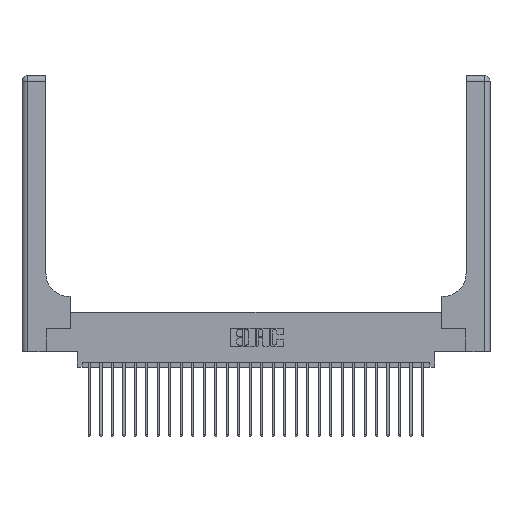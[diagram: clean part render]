
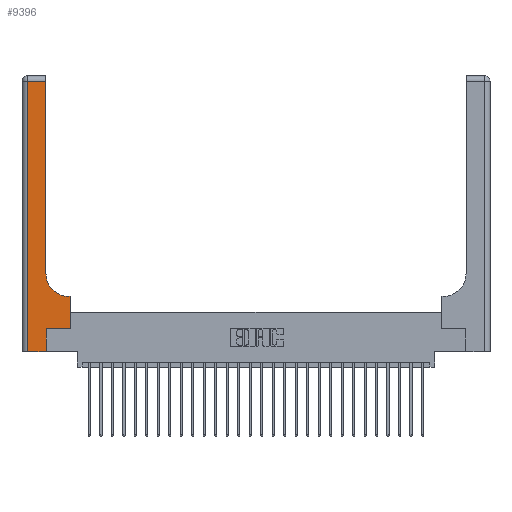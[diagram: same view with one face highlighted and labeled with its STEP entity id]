
A CAD part, top view. The second image highlights one B-rep face of the part: STEP entity #9396.
In plain terms, the highlighted planar face has unit normal (0, 0, 1).
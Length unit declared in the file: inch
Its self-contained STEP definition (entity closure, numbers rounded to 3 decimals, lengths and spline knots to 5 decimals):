
#610 = LINE ( 'NONE', #25601, #19397 ) ;
#848 = CARTESIAN_POINT ( 'NONE',  ( 0., 2.94, 0.37 ) ) ;
#2397 = FACE_OUTER_BOUND ( 'NONE', #11196, .T. ) ;
#2480 = ORIENTED_EDGE ( 'NONE', *, *, #14184, .T. ) ;
#3063 = LINE ( 'NONE', #21761, #20625 ) ;
#3380 = VECTOR ( 'NONE', #16732, 39.37008 ) ;
#3542 = DIRECTION ( 'NONE',  ( -1., 0., 0. ) ) ;
#4198 = CARTESIAN_POINT ( 'NONE',  ( 0.51, 0.85, 0.37 ) ) ;
#5097 = LINE ( 'NONE', #848, #18580 ) ;
#5591 = LINE ( 'NONE', #11713, #22896 ) ;
#5715 = DIRECTION ( 'NONE',  ( 0., 0., -1. ) ) ;
#6107 = LINE ( 'NONE', #14394, #15006 ) ;
#6424 = LINE ( 'NONE', #10770, #21570 ) ;
#7091 = EDGE_CURVE ( 'NONE', #9971, #16567, #6424, .T. ) ;
#7911 = DIRECTION ( 'NONE',  ( 0., 0., -1. ) ) ;
#8408 = EDGE_CURVE ( 'NONE', #21682, #12638, #18558, .T. ) ;
#8945 = CARTESIAN_POINT ( 'NONE',  ( 0.26, 2.94, 0.37 ) ) ;
#9205 = DIRECTION ( 'NONE',  ( 0., 1., 0. ) ) ;
#9396 = ADVANCED_FACE ( 'NONE', ( #2397 ), #26597, .F. ) ;
#9971 = VERTEX_POINT ( 'NONE', #10912 ) ;
#10157 = ORIENTED_EDGE ( 'NONE', *, *, #7091, .T. ) ;
#10770 = CARTESIAN_POINT ( 'NONE',  ( 0.265, 0.25, 0.37 ) ) ;
#10912 = CARTESIAN_POINT ( 'NONE',  ( 0.265, 0.25, 0.37 ) ) ;
#11063 = DIRECTION ( 'NONE',  ( 0., 1., 0. ) ) ;
#11196 = EDGE_LOOP ( 'NONE', ( #14024, #17132, #2480, #25426, #21417, #10157, #21646, #14315, #12324 ) ) ;
#11713 = CARTESIAN_POINT ( 'NONE',  ( 0.528, 0.25, 0.37 ) ) ;
#12040 = EDGE_CURVE ( 'NONE', #22289, #9971, #610, .T. ) ;
#12127 = AXIS2_PLACEMENT_3D ( 'NONE', #22630, #7911, #16191 ) ;
#12324 = ORIENTED_EDGE ( 'NONE', *, *, #19884, .T. ) ;
#12563 = VERTEX_POINT ( 'NONE', #15205 ) ;
#12638 = VERTEX_POINT ( 'NONE', #8945 ) ;
#12974 = DIRECTION ( 'NONE',  ( 1., 0., 0. ) ) ;
#13153 = AXIS2_PLACEMENT_3D ( 'NONE', #4198, #5715, #16312 ) ;
#14024 = ORIENTED_EDGE ( 'NONE', *, *, #8408, .T. ) ;
#14184 = EDGE_CURVE ( 'NONE', #16654, #19240, #15310, .T. ) ;
#14315 = ORIENTED_EDGE ( 'NONE', *, *, #16786, .T. ) ;
#14380 = VERTEX_POINT ( 'NONE', #22413 ) ;
#14394 = CARTESIAN_POINT ( 'NONE',  ( 0.26, 0.6, 0.37 ) ) ;
#14618 = EDGE_CURVE ( 'NONE', #12638, #16654, #5097, .T. ) ;
#14637 = EDGE_CURVE ( 'NONE', #16567, #14380, #5591, .T. ) ;
#14658 = DIRECTION ( 'NONE',  ( -1., 0., 0. ) ) ;
#14885 = CIRCLE ( 'NONE', #13153, 0.25 ) ;
#15006 = VECTOR ( 'NONE', #14658, 39.37008 ) ;
#15205 = CARTESIAN_POINT ( 'NONE',  ( 0.51, 0.6, 0.37 ) ) ;
#15310 = LINE ( 'NONE', #19569, #17673 ) ;
#16191 = DIRECTION ( 'NONE',  ( -1., 0., 0. ) ) ;
#16312 = DIRECTION ( 'NONE',  ( 1., 0., 0. ) ) ;
#16567 = VERTEX_POINT ( 'NONE', #26576 ) ;
#16654 = VERTEX_POINT ( 'NONE', #19923 ) ;
#16732 = DIRECTION ( 'NONE',  ( 0., 1., 0. ) ) ;
#16786 = EDGE_CURVE ( 'NONE', #14380, #12563, #6107, .T. ) ;
#17132 = ORIENTED_EDGE ( 'NONE', *, *, #14618, .T. ) ;
#17293 = CARTESIAN_POINT ( 'NONE',  ( 0.265, 0., 0.37 ) ) ;
#17673 = VECTOR ( 'NONE', #19716, 39.37008 ) ;
#18558 = LINE ( 'NONE', #20617, #3380 ) ;
#18580 = VECTOR ( 'NONE', #3542, 39.37008 ) ;
#18589 = CARTESIAN_POINT ( 'NONE',  ( 0.26, 0.85, 0.37 ) ) ;
#19240 = VERTEX_POINT ( 'NONE', #20099 ) ;
#19397 = VECTOR ( 'NONE', #9205, 39.37008 ) ;
#19569 = CARTESIAN_POINT ( 'NONE',  ( 0.06, 3., 0.37 ) ) ;
#19716 = DIRECTION ( 'NONE',  ( 0., -1., 0. ) ) ;
#19884 = EDGE_CURVE ( 'NONE', #12563, #21682, #14885, .T. ) ;
#19923 = CARTESIAN_POINT ( 'NONE',  ( 0.06, 2.94, 0.37 ) ) ;
#20099 = CARTESIAN_POINT ( 'NONE',  ( 0.06, 0., 0.37 ) ) ;
#20617 = CARTESIAN_POINT ( 'NONE',  ( 0.26, 3., 0.37 ) ) ;
#20625 = VECTOR ( 'NONE', #12974, 39.37008 ) ;
#21301 = EDGE_CURVE ( 'NONE', #19240, #22289, #3063, .T. ) ;
#21417 = ORIENTED_EDGE ( 'NONE', *, *, #12040, .T. ) ;
#21570 = VECTOR ( 'NONE', #22786, 39.37008 ) ;
#21646 = ORIENTED_EDGE ( 'NONE', *, *, #14637, .T. ) ;
#21682 = VERTEX_POINT ( 'NONE', #18589 ) ;
#21761 = CARTESIAN_POINT ( 'NONE',  ( 0., 0., 0.37 ) ) ;
#22289 = VERTEX_POINT ( 'NONE', #17293 ) ;
#22413 = CARTESIAN_POINT ( 'NONE',  ( 0.528, 0.6, 0.37 ) ) ;
#22630 = CARTESIAN_POINT ( 'NONE',  ( 0., 3., 0.37 ) ) ;
#22786 = DIRECTION ( 'NONE',  ( 1., 0., 0. ) ) ;
#22896 = VECTOR ( 'NONE', #11063, 39.37008 ) ;
#25426 = ORIENTED_EDGE ( 'NONE', *, *, #21301, .T. ) ;
#25601 = CARTESIAN_POINT ( 'NONE',  ( 0.265, 0., 0.37 ) ) ;
#26576 = CARTESIAN_POINT ( 'NONE',  ( 0.528, 0.25, 0.37 ) ) ;
#26597 = PLANE ( 'NONE',  #12127 ) ;
